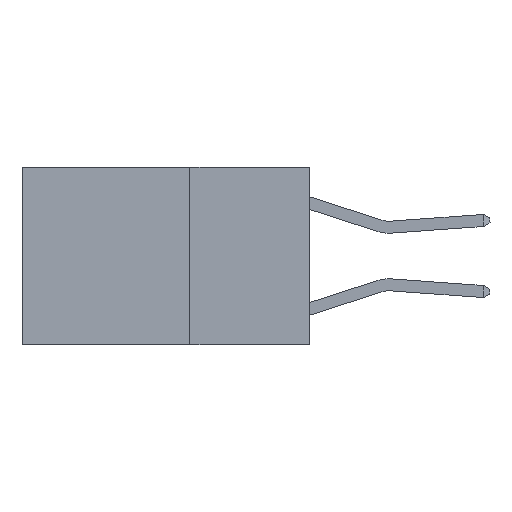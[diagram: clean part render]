
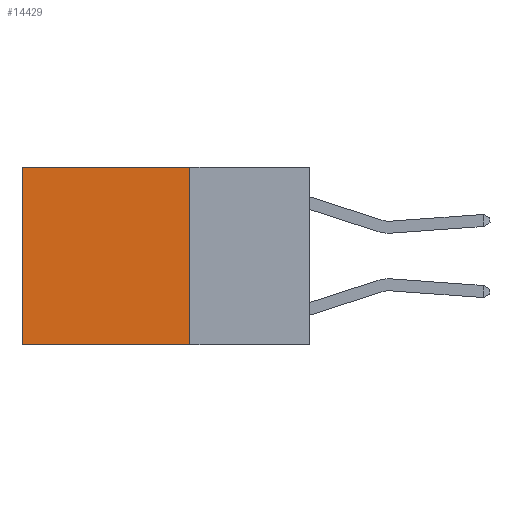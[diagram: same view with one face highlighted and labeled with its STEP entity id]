
A CAD part, left-side view. The second image highlights one B-rep face of the part: STEP entity #14429.
In plain terms, the highlighted planar face has unit normal (-1, 0, 0).
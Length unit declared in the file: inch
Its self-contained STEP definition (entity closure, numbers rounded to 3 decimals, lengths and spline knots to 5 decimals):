
#1155 = CARTESIAN_POINT ( 'NONE',  ( 0.2625, 0.6, 0. ) ) ;
#1676 = LINE ( 'NONE', #11306, #6255 ) ;
#2276 = VECTOR ( 'NONE', #8151, 39.37008 ) ;
#2694 = FACE_OUTER_BOUND ( 'NONE', #14452, .T. ) ;
#2949 = DIRECTION ( 'NONE',  ( 0., 0., -1. ) ) ;
#4689 = LINE ( 'NONE', #18775, #13422 ) ;
#4710 = EDGE_CURVE ( 'NONE', #5353, #13528, #10963, .T. ) ;
#5353 = VERTEX_POINT ( 'NONE', #1155 ) ;
#6000 = CARTESIAN_POINT ( 'NONE',  ( 0.2625, 0.25, 0. ) ) ;
#6255 = VECTOR ( 'NONE', #16556, 39.37008 ) ;
#6660 = ORIENTED_EDGE ( 'NONE', *, *, #16079, .F. ) ;
#8151 = DIRECTION ( 'NONE',  ( 0., 0., -1. ) ) ;
#8667 = LINE ( 'NONE', #6000, #12766 ) ;
#9483 = CARTESIAN_POINT ( 'NONE',  ( 0.2625, 0.25, -0.37 ) ) ;
#10890 = CARTESIAN_POINT ( 'NONE',  ( 0.2625, 0.6, -0.37 ) ) ;
#10927 = EDGE_CURVE ( 'NONE', #12567, #5353, #8667, .T. ) ;
#10963 = LINE ( 'NONE', #13361, #2276 ) ;
#11306 = CARTESIAN_POINT ( 'NONE',  ( 0.2625, 0.25, -0.37 ) ) ;
#11617 = CARTESIAN_POINT ( 'NONE',  ( 0.2625, 0.25, 0. ) ) ;
#11622 = ORIENTED_EDGE ( 'NONE', *, *, #4710, .T. ) ;
#11747 = ORIENTED_EDGE ( 'NONE', *, *, #15232, .F. ) ;
#11763 = CARTESIAN_POINT ( 'NONE',  ( 0.2625, 0.25, 0. ) ) ;
#11973 = DIRECTION ( 'NONE',  ( 0., 0., -1. ) ) ;
#12567 = VERTEX_POINT ( 'NONE', #11763 ) ;
#12766 = VECTOR ( 'NONE', #12968, 39.37008 ) ;
#12968 = DIRECTION ( 'NONE',  ( 0., 1., 0. ) ) ;
#13361 = CARTESIAN_POINT ( 'NONE',  ( 0.2625, 0.6, 0. ) ) ;
#13378 = DIRECTION ( 'NONE',  ( 1., 0., 0. ) ) ;
#13422 = VECTOR ( 'NONE', #11973, 39.37008 ) ;
#13528 = VERTEX_POINT ( 'NONE', #10890 ) ;
#14429 = ADVANCED_FACE ( 'NONE', ( #2694 ), #22013, .F. ) ;
#14452 = EDGE_LOOP ( 'NONE', ( #11622, #6660, #11747, #21769 ) ) ;
#15232 = EDGE_CURVE ( 'NONE', #12567, #21770, #4689, .T. ) ;
#16079 = EDGE_CURVE ( 'NONE', #21770, #13528, #1676, .T. ) ;
#16556 = DIRECTION ( 'NONE',  ( 0., 1., 0. ) ) ;
#17237 = AXIS2_PLACEMENT_3D ( 'NONE', #11617, #13378, #2949 ) ;
#18775 = CARTESIAN_POINT ( 'NONE',  ( 0.2625, 0.25, 0. ) ) ;
#21769 = ORIENTED_EDGE ( 'NONE', *, *, #10927, .T. ) ;
#21770 = VERTEX_POINT ( 'NONE', #9483 ) ;
#22013 = PLANE ( 'NONE',  #17237 ) ;
